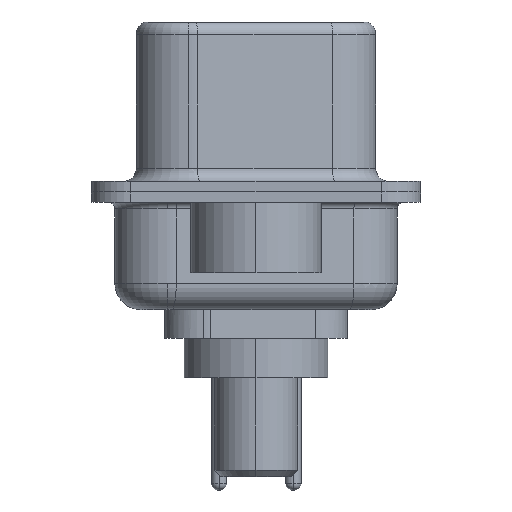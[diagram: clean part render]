
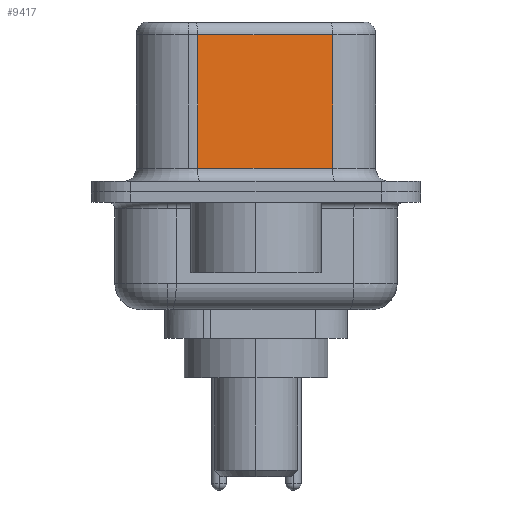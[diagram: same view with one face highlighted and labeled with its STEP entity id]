
A CAD part, left-side view. The second image highlights one B-rep face of the part: STEP entity #9417.
In plain terms, the highlighted planar face has unit normal (-0.985, -0.174, 0).
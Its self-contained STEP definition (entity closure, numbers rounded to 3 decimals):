
#76 = CARTESIAN_POINT ( 'NONE',  ( 3.655, 2.233, 6.02 ) ) ;
#383 = VERTEX_POINT ( 'NONE', #6796 ) ;
#669 = LINE ( 'NONE', #11622, #12862 ) ;
#1126 = CARTESIAN_POINT ( 'NONE',  ( 4.565, -2.927, 6.02 ) ) ;
#1185 = DIRECTION ( 'NONE',  ( -0.174, 0.985, 0. ) ) ;
#1756 = CARTESIAN_POINT ( 'NONE',  ( 4.565, -2.927, 0.9 ) ) ;
#2035 = VECTOR ( 'NONE', #1185, 1000. ) ;
#2337 = ORIENTED_EDGE ( 'NONE', *, *, #5571, .F. ) ;
#2370 = VECTOR ( 'NONE', #11916, 1000. ) ;
#2401 = ORIENTED_EDGE ( 'NONE', *, *, #5484, .T. ) ;
#2441 = LINE ( 'NONE', #1126, #2035 ) ;
#3348 = DIRECTION ( 'NONE',  ( 0.174, -0.985, 0. ) ) ;
#5307 = VECTOR ( 'NONE', #3348, 1000. ) ;
#5328 = DIRECTION ( 'NONE',  ( -0.174, 0.985, 0. ) ) ;
#5484 = EDGE_CURVE ( 'NONE', #8923, #383, #669, .T. ) ;
#5571 = EDGE_CURVE ( 'NONE', #14107, #9358, #9106, .T. ) ;
#5579 = EDGE_CURVE ( 'NONE', #383, #9358, #12143, .T. ) ;
#6796 = CARTESIAN_POINT ( 'NONE',  ( 3.655, 2.233, 0.9 ) ) ;
#8923 = VERTEX_POINT ( 'NONE', #76 ) ;
#9106 = LINE ( 'NONE', #12052, #2370 ) ;
#9120 = CARTESIAN_POINT ( 'NONE',  ( 4.565, -2.927, 6.52 ) ) ;
#9358 = VERTEX_POINT ( 'NONE', #13350 ) ;
#9417 = ADVANCED_FACE ( 'NONE', ( #9735 ), #14797, .F. ) ;
#9735 = FACE_OUTER_BOUND ( 'NONE', #13181, .T. ) ;
#9763 = EDGE_CURVE ( 'NONE', #14107, #8923, #2441, .T. ) ;
#11622 = CARTESIAN_POINT ( 'NONE',  ( 3.655, 2.233, 6.52 ) ) ;
#11916 = DIRECTION ( 'NONE',  ( 0., 0., -1. ) ) ;
#12052 = CARTESIAN_POINT ( 'NONE',  ( 4.565, -2.927, 6.52 ) ) ;
#12143 = LINE ( 'NONE', #1756, #5307 ) ;
#12333 = ORIENTED_EDGE ( 'NONE', *, *, #5579, .T. ) ;
#12558 = DIRECTION ( 'NONE',  ( 0.985, 0.174, 0. ) ) ;
#12602 = DIRECTION ( 'NONE',  ( 0., 0., -1. ) ) ;
#12862 = VECTOR ( 'NONE', #12602, 1000. ) ;
#13159 = ORIENTED_EDGE ( 'NONE', *, *, #9763, .T. ) ;
#13181 = EDGE_LOOP ( 'NONE', ( #2337, #13159, #2401, #12333 ) ) ;
#13300 = AXIS2_PLACEMENT_3D ( 'NONE', #9120, #12558, #5328 ) ;
#13350 = CARTESIAN_POINT ( 'NONE',  ( 4.565, -2.927, 0.9 ) ) ;
#14030 = CARTESIAN_POINT ( 'NONE',  ( 4.565, -2.927, 6.02 ) ) ;
#14107 = VERTEX_POINT ( 'NONE', #14030 ) ;
#14797 = PLANE ( 'NONE',  #13300 ) ;
